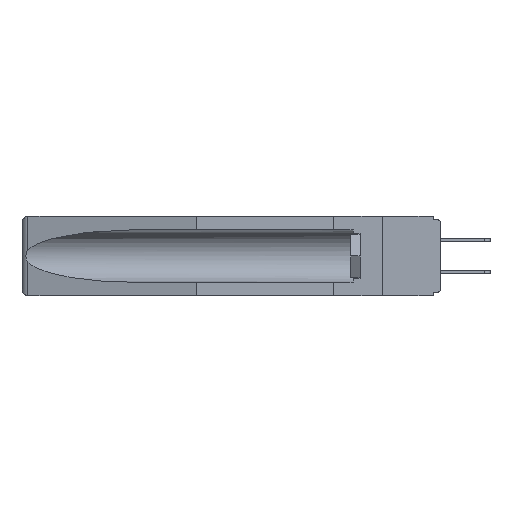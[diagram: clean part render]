
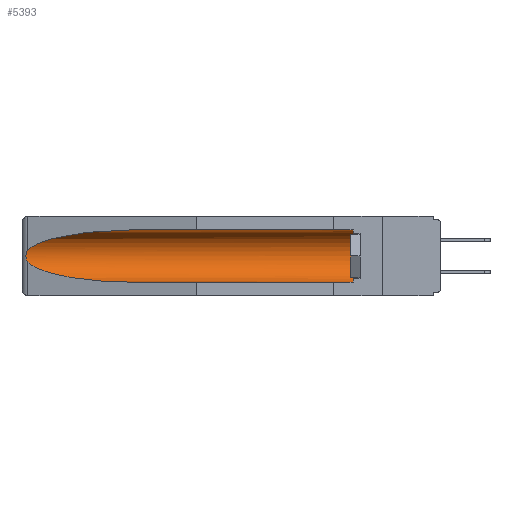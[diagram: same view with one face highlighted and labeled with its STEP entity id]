
A CAD part, left-side view. The second image highlights one B-rep face of the part: STEP entity #5393.
In plain terms, the highlighted cylindrical face has radius 2.857 mm (diameter 5.715 mm), a partial arc.
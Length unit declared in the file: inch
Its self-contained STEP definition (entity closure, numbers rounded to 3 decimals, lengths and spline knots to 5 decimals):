
#375 = VERTEX_POINT ( 'NONE', #20606 ) ;
#869 = EDGE_LOOP ( 'NONE', ( #8542, #18772, #10737, #7196, #17674, #14756 ) ) ;
#1314 = EDGE_CURVE ( 'NONE', #5838, #375, #22317, .T. ) ;
#1340 = CARTESIAN_POINT ( 'NONE',  ( 0.26654, 1.53092, -0.15636 ) ) ;
#1425 = CARTESIAN_POINT ( 'NONE',  ( 0.26537, 1.52718, -0.19328 ) ) ;
#1474 = VECTOR ( 'NONE', #3659, 39.37008 ) ;
#1510 = CARTESIAN_POINT ( 'NONE',  ( 0.155, 1.07973, -0.059 ) ) ;
#2612 = CARTESIAN_POINT ( 'NONE',  ( 0.155, 1.07973, -0.059 ) ) ;
#3310 = CARTESIAN_POINT ( 'NONE',  ( 0.155, -0.30754, -0.059 ) ) ;
#3461 = DIRECTION ( 'NONE',  ( 0., 1., 0. ) ) ;
#3659 = DIRECTION ( 'NONE',  ( 0., 1., 0. ) ) ;
#4186 = LINE ( 'NONE', #7623, #1474 ) ;
#4846 = B_SPLINE_CURVE_WITH_KNOTS ( 'NONE', 3,
 ( #12901, #16676, #1340, #9100, #22240, #18399, #18583, #6856, #7197, #1425 ),
 .UNSPECIFIED., .F., .F.,
 ( 4, 2, 2, 2, 4 ),
 ( 0., 0.00029, 0.00058, 0.00087, 0.00117 ),
 .UNSPECIFIED. ) ;
#5173 = CARTESIAN_POINT ( 'NONE',  ( 0.26537, 1.52718, -0.19328 ) ) ;
#5302 = CARTESIAN_POINT ( 'NONE',  ( 0.21114, 1.30732, -0.059 ) ) ;
#5393 = ADVANCED_FACE ( 'NONE', ( #8507 ), #17736, .F. ) ;
#5436 = CARTESIAN_POINT ( 'NONE',  ( 0.25451, 1.48313, -0.24835 ) ) ;
#5472 = DIRECTION ( 'NONE',  ( 0., 0., 1. ) ) ;
#5838 = VERTEX_POINT ( 'NONE', #13845 ) ;
#6856 = CARTESIAN_POINT ( 'NONE',  ( 0.26655, 1.53094, -0.18657 ) ) ;
#7061 = CARTESIAN_POINT ( 'NONE',  ( 0.155, 1.07973, -0.284 ) ) ;
#7196 = ORIENTED_EDGE ( 'NONE', *, *, #17039, .F. ) ;
#7197 = CARTESIAN_POINT ( 'NONE',  ( 0.26597, 1.5296, -0.19026 ) ) ;
#7486 = VERTEX_POINT ( 'NONE', #13103 ) ;
#7623 = CARTESIAN_POINT ( 'NONE',  ( 0.155, -0.30754, -0.284 ) ) ;
#7870 = VERTEX_POINT ( 'NONE', #21235 ) ;
#8507 = FACE_OUTER_BOUND ( 'NONE', #869, .T. ) ;
#8542 = ORIENTED_EDGE ( 'NONE', *, *, #22146, .T. ) ;
#8852 = CARTESIAN_POINT ( 'NONE',  ( 0.155, 0.126, -0.1715 ) ) ;
#9100 = CARTESIAN_POINT ( 'NONE',  ( 0.2673, 1.5327, -0.16383 ) ) ;
#9579 = EDGE_CURVE ( 'NONE', #21752, #7486, #4846, .T. ) ;
#10105 = EDGE_CURVE ( 'NONE', #375, #10476, #16854, .T. ) ;
#10476 = VERTEX_POINT ( 'NONE', #2612 ) ;
#10686 =( BOUNDED_CURVE ( )  B_SPLINE_CURVE ( 3, ( #1510, #5302, #14913, #22307 ),
 .UNSPECIFIED., .F., .T. ) 
 B_SPLINE_CURVE_WITH_KNOTS ( ( 4, 4 ),
 ( 4.71239, 6.08839 ),
 .UNSPECIFIED. ) 
 CURVE ( )  GEOMETRIC_REPRESENTATION_ITEM ( )  RATIONAL_B_SPLINE_CURVE ( ( 1., 0.848, 0.848, 1. ) ) 
 REPRESENTATION_ITEM ( '' )  );
#10737 = ORIENTED_EDGE ( 'NONE', *, *, #11400, .T. ) ;
#11400 = EDGE_CURVE ( 'NONE', #7486, #7870, #19568, .T. ) ;
#12901 = CARTESIAN_POINT ( 'NONE',  ( 0.26537, 1.52718, -0.14972 ) ) ;
#13103 = CARTESIAN_POINT ( 'NONE',  ( 0.26537, 1.52718, -0.19328 ) ) ;
#13256 = CARTESIAN_POINT ( 'NONE',  ( 0.155, -0.30754, -0.1715 ) ) ;
#13845 = CARTESIAN_POINT ( 'NONE',  ( 0.155, 0.126, -0.284 ) ) ;
#14756 = ORIENTED_EDGE ( 'NONE', *, *, #10105, .T. ) ;
#14913 = CARTESIAN_POINT ( 'NONE',  ( 0.25451, 1.48313, -0.09465 ) ) ;
#15088 = DIRECTION ( 'NONE',  ( 0., 1., 0. ) ) ;
#16158 = AXIS2_PLACEMENT_3D ( 'NONE', #8852, #20424, #22170 ) ;
#16676 = CARTESIAN_POINT ( 'NONE',  ( 0.26597, 1.52961, -0.15275 ) ) ;
#16854 = LINE ( 'NONE', #3310, #24590 ) ;
#17039 = EDGE_CURVE ( 'NONE', #5838, #7870, #4186, .T. ) ;
#17674 = ORIENTED_EDGE ( 'NONE', *, *, #1314, .T. ) ;
#17736 = CYLINDRICAL_SURFACE ( 'NONE', #24349, 0.1125 ) ;
#18399 = CARTESIAN_POINT ( 'NONE',  ( 0.2675, 1.53308, -0.17534 ) ) ;
#18583 = CARTESIAN_POINT ( 'NONE',  ( 0.2673, 1.53269, -0.17917 ) ) ;
#18772 = ORIENTED_EDGE ( 'NONE', *, *, #9579, .T. ) ;
#19568 =( BOUNDED_CURVE ( )  B_SPLINE_CURVE ( 3, ( #5173, #5436, #20443, #7061 ),
 .UNSPECIFIED., .F., .F. ) 
 B_SPLINE_CURVE_WITH_KNOTS ( ( 4, 4 ),
 ( 0.1948, 1.5708 ),
 .UNSPECIFIED. ) 
 CURVE ( )  GEOMETRIC_REPRESENTATION_ITEM ( )  RATIONAL_B_SPLINE_CURVE ( ( 1., 0.848, 0.848, 1. ) ) 
 REPRESENTATION_ITEM ( '' )  );
#20424 = DIRECTION ( 'NONE',  ( 0., -1., 0. ) ) ;
#20443 = CARTESIAN_POINT ( 'NONE',  ( 0.21114, 1.30732, -0.284 ) ) ;
#20606 = CARTESIAN_POINT ( 'NONE',  ( 0.155, 0.126, -0.059 ) ) ;
#21235 = CARTESIAN_POINT ( 'NONE',  ( 0.155, 1.07973, -0.284 ) ) ;
#21752 = VERTEX_POINT ( 'NONE', #23370 ) ;
#22146 = EDGE_CURVE ( 'NONE', #10476, #21752, #10686, .T. ) ;
#22170 = DIRECTION ( 'NONE',  ( 0., 0., 1. ) ) ;
#22240 = CARTESIAN_POINT ( 'NONE',  ( 0.2675, 1.53308, -0.16763 ) ) ;
#22307 = CARTESIAN_POINT ( 'NONE',  ( 0.26537, 1.52718, -0.14972 ) ) ;
#22317 = CIRCLE ( 'NONE', #16158, 0.1125 ) ;
#23370 = CARTESIAN_POINT ( 'NONE',  ( 0.26537, 1.52718, -0.14972 ) ) ;
#24349 = AXIS2_PLACEMENT_3D ( 'NONE', #13256, #3461, #5472 ) ;
#24590 = VECTOR ( 'NONE', #15088, 39.37008 ) ;
